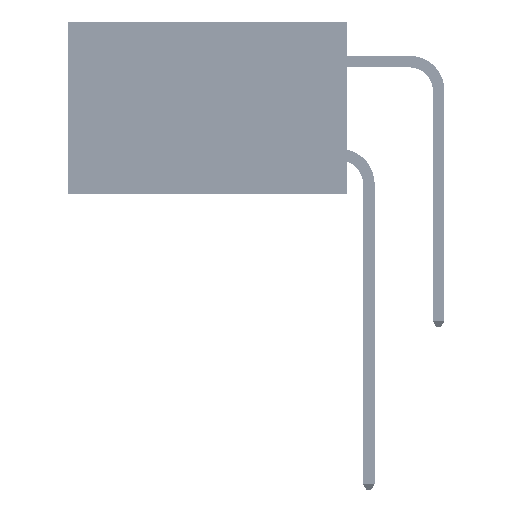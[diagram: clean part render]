
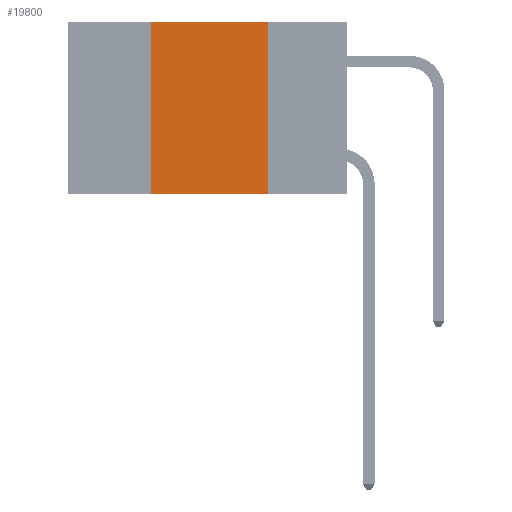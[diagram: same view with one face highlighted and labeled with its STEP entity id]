
A CAD part, left-side view. The second image highlights one B-rep face of the part: STEP entity #19800.
In plain terms, the highlighted planar face has unit normal (-1, 0, 0).
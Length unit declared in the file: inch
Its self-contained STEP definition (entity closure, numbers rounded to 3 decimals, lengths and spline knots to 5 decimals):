
#50 = ORIENTED_EDGE ( 'NONE', *, *, #6199, .F. ) ;
#1450 = CARTESIAN_POINT ( 'NONE',  ( 0., 0.6, 0. ) ) ;
#5281 = CARTESIAN_POINT ( 'NONE',  ( 0., 0.42, -0.37 ) ) ;
#6138 = LINE ( 'NONE', #30209, #41176 ) ;
#6199 = EDGE_CURVE ( 'NONE', #34438, #14543, #26740, .T. ) ;
#7462 = EDGE_LOOP ( 'NONE', ( #13895, #12851, #50, #14754 ) ) ;
#8233 = CARTESIAN_POINT ( 'NONE',  ( 0., 0.42, 0. ) ) ;
#10436 = LINE ( 'NONE', #16378, #49783 ) ;
#10891 = VECTOR ( 'NONE', #38921, 39.37008 ) ;
#12851 = ORIENTED_EDGE ( 'NONE', *, *, #34516, .F. ) ;
#13623 = LINE ( 'NONE', #1450, #33469 ) ;
#13818 = VERTEX_POINT ( 'NONE', #14659 ) ;
#13895 = ORIENTED_EDGE ( 'NONE', *, *, #33655, .F. ) ;
#13899 = DIRECTION ( 'NONE',  ( 1., 0., 0. ) ) ;
#14139 = FACE_OUTER_BOUND ( 'NONE', #7462, .T. ) ;
#14162 = VERTEX_POINT ( 'NONE', #25262 ) ;
#14543 = VERTEX_POINT ( 'NONE', #33335 ) ;
#14659 = CARTESIAN_POINT ( 'NONE',  ( 0., 0.17, -0.37 ) ) ;
#14754 = ORIENTED_EDGE ( 'NONE', *, *, #23758, .T. ) ;
#16378 = CARTESIAN_POINT ( 'NONE',  ( 0., 0.17, 0. ) ) ;
#16932 = DIRECTION ( 'NONE',  ( 0., -1., 0. ) ) ;
#19800 = ADVANCED_FACE ( 'NONE', ( #14139 ), #21018, .F. ) ;
#21018 = PLANE ( 'NONE',  #21063 ) ;
#21063 = AXIS2_PLACEMENT_3D ( 'NONE', #41290, #13899, #40290 ) ;
#23758 = EDGE_CURVE ( 'NONE', #34438, #13818, #6138, .T. ) ;
#25262 = CARTESIAN_POINT ( 'NONE',  ( 0., 0.17, 0. ) ) ;
#26740 = LINE ( 'NONE', #8233, #10891 ) ;
#30209 = CARTESIAN_POINT ( 'NONE',  ( 0., 0.6, -0.37 ) ) ;
#33335 = CARTESIAN_POINT ( 'NONE',  ( 0., 0.42, 0. ) ) ;
#33469 = VECTOR ( 'NONE', #16932, 39.37008 ) ;
#33655 = EDGE_CURVE ( 'NONE', #14162, #13818, #10436, .T. ) ;
#34438 = VERTEX_POINT ( 'NONE', #5281 ) ;
#34516 = EDGE_CURVE ( 'NONE', #14543, #14162, #13623, .T. ) ;
#38921 = DIRECTION ( 'NONE',  ( 0., 0., 1. ) ) ;
#40290 = DIRECTION ( 'NONE',  ( 0., 0., -1. ) ) ;
#41176 = VECTOR ( 'NONE', #49251, 39.37008 ) ;
#41290 = CARTESIAN_POINT ( 'NONE',  ( 0., 0.6, 0. ) ) ;
#47349 = DIRECTION ( 'NONE',  ( 0., 0., -1. ) ) ;
#49251 = DIRECTION ( 'NONE',  ( 0., -1., 0. ) ) ;
#49783 = VECTOR ( 'NONE', #47349, 39.37008 ) ;
